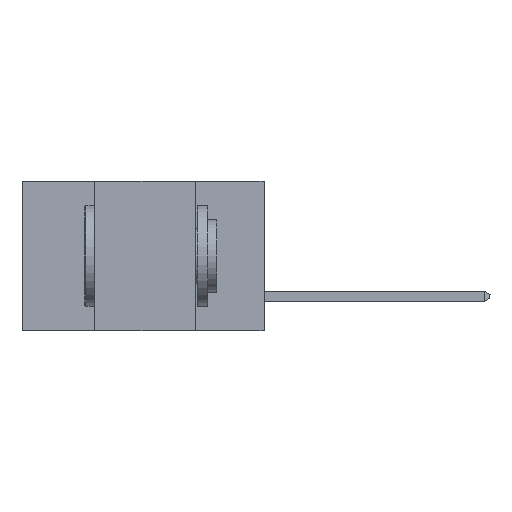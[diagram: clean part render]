
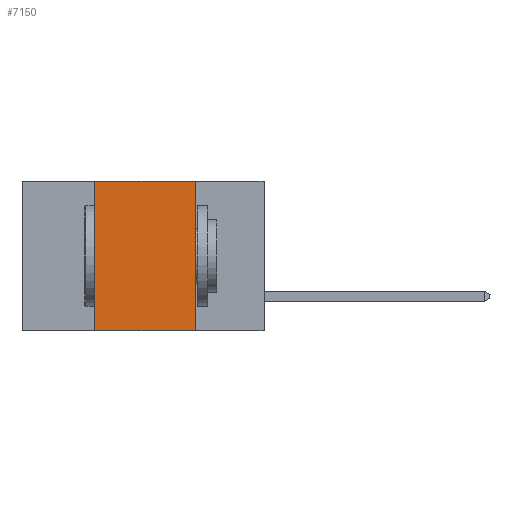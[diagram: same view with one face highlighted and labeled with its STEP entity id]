
A CAD part, left-side view. The second image highlights one B-rep face of the part: STEP entity #7150.
In plain terms, the highlighted planar face has unit normal (-1, 0, 0).
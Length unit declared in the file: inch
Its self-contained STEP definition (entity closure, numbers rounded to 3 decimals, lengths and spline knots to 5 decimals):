
#1322 = ORIENTED_EDGE ( 'NONE', *, *, #4270, .F. ) ;
#1362 = AXIS2_PLACEMENT_3D ( 'NONE', #9565, #13291, #5761 ) ;
#1784 = EDGE_CURVE ( 'NONE', #7276, #10100, #3346, .T. ) ;
#1795 = CARTESIAN_POINT ( 'NONE',  ( 0., 0.6, 0. ) ) ;
#2415 = EDGE_LOOP ( 'NONE', ( #1322, #2979, #9511, #10160 ) ) ;
#2623 = DIRECTION ( 'NONE',  ( 0., -1., 0. ) ) ;
#2979 = ORIENTED_EDGE ( 'NONE', *, *, #1784, .F. ) ;
#3239 = CARTESIAN_POINT ( 'NONE',  ( 0., 0.17, 0. ) ) ;
#3346 = LINE ( 'NONE', #1795, #6999 ) ;
#3797 = CARTESIAN_POINT ( 'NONE',  ( 0., 0.17, -0.37 ) ) ;
#4270 = EDGE_CURVE ( 'NONE', #10100, #12137, #8219, .T. ) ;
#4604 = PLANE ( 'NONE',  #1362 ) ;
#4826 = VECTOR ( 'NONE', #6124, 39.37008 ) ;
#5761 = DIRECTION ( 'NONE',  ( 0., 0., -1. ) ) ;
#6124 = DIRECTION ( 'NONE',  ( 0., 0., 1. ) ) ;
#6827 = DIRECTION ( 'NONE',  ( 0., -1., 0. ) ) ;
#6832 = CARTESIAN_POINT ( 'NONE',  ( 0., 0.17, -0.37 ) ) ;
#6999 = VECTOR ( 'NONE', #6827, 39.37008 ) ;
#7150 = ADVANCED_FACE ( 'NONE', ( #14624 ), #4604, .F. ) ;
#7276 = VERTEX_POINT ( 'NONE', #14546 ) ;
#7376 = CARTESIAN_POINT ( 'NONE',  ( 0., 0.42, -0.37 ) ) ;
#7720 = LINE ( 'NONE', #10234, #10355 ) ;
#8219 = LINE ( 'NONE', #6832, #15725 ) ;
#9308 = DIRECTION ( 'NONE',  ( 0., 0., -1. ) ) ;
#9511 = ORIENTED_EDGE ( 'NONE', *, *, #11564, .F. ) ;
#9565 = CARTESIAN_POINT ( 'NONE',  ( 0., 0.6, 0. ) ) ;
#10100 = VERTEX_POINT ( 'NONE', #3239 ) ;
#10160 = ORIENTED_EDGE ( 'NONE', *, *, #14866, .T. ) ;
#10234 = CARTESIAN_POINT ( 'NONE',  ( 0., 0.6, -0.37 ) ) ;
#10355 = VECTOR ( 'NONE', #2623, 39.37008 ) ;
#11564 = EDGE_CURVE ( 'NONE', #12253, #7276, #15902, .T. ) ;
#12137 = VERTEX_POINT ( 'NONE', #3797 ) ;
#12253 = VERTEX_POINT ( 'NONE', #12968 ) ;
#12968 = CARTESIAN_POINT ( 'NONE',  ( 0., 0.42, -0.37 ) ) ;
#13291 = DIRECTION ( 'NONE',  ( 1., 0., 0. ) ) ;
#14546 = CARTESIAN_POINT ( 'NONE',  ( 0., 0.42, 0. ) ) ;
#14624 = FACE_OUTER_BOUND ( 'NONE', #2415, .T. ) ;
#14866 = EDGE_CURVE ( 'NONE', #12253, #12137, #7720, .T. ) ;
#15725 = VECTOR ( 'NONE', #9308, 39.37008 ) ;
#15902 = LINE ( 'NONE', #7376, #4826 ) ;
